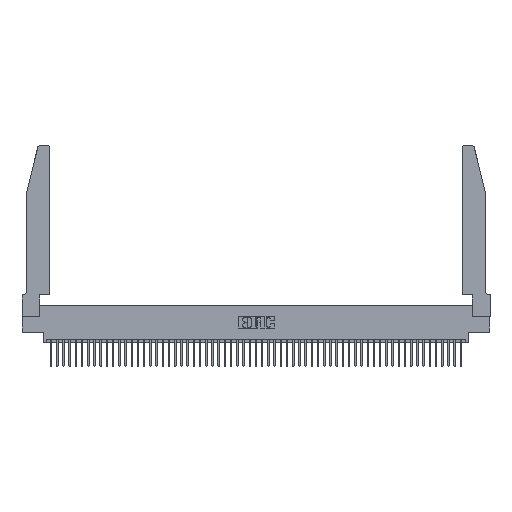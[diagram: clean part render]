
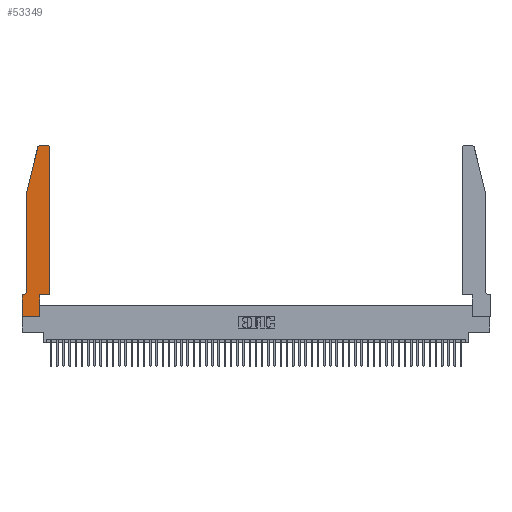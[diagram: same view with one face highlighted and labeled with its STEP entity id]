
A CAD part, top view. The second image highlights one B-rep face of the part: STEP entity #53349.
In plain terms, the highlighted planar face has unit normal (0, 0, 1).
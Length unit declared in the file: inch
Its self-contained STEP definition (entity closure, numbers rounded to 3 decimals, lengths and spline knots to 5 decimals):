
#798 = VECTOR ( 'NONE', #17286, 39.37008 ) ;
#1004 = LINE ( 'NONE', #35745, #33051 ) ;
#1583 = DIRECTION ( 'NONE',  ( -1., 0., 0. ) ) ;
#1916 = DIRECTION ( 'NONE',  ( -1., 0., 0. ) ) ;
#2500 = CARTESIAN_POINT ( 'NONE',  ( 0.4205, 2.72, 0.37 ) ) ;
#2625 = ORIENTED_EDGE ( 'NONE', *, *, #51947, .T. ) ;
#2763 = DIRECTION ( 'NONE',  ( 0., -1., 0. ) ) ;
#2934 = LINE ( 'NONE', #49160, #19914 ) ;
#3525 = VERTEX_POINT ( 'NONE', #50909 ) ;
#4084 = CARTESIAN_POINT ( 'NONE',  ( 0.4505, 0.35, 0.37 ) ) ;
#4349 = CARTESIAN_POINT ( 'NONE',  ( 0., 0., 0.37 ) ) ;
#5816 = VECTOR ( 'NONE', #54023, 39.37008 ) ;
#6450 = VERTEX_POINT ( 'NONE', #38576 ) ;
#6596 = CARTESIAN_POINT ( 'NONE',  ( 0., 0., 0.37 ) ) ;
#6844 = VERTEX_POINT ( 'NONE', #53510 ) ;
#7007 = VERTEX_POINT ( 'NONE', #29158 ) ;
#7315 = CARTESIAN_POINT ( 'NONE',  ( 0.0055, 0.35, 0.37 ) ) ;
#8256 = DIRECTION ( 'NONE',  ( 1., 0., 0. ) ) ;
#8524 = DIRECTION ( 'NONE',  ( 1., 0., 0. ) ) ;
#9118 = VECTOR ( 'NONE', #2763, 39.37008 ) ;
#9578 = PLANE ( 'NONE',  #10387 ) ;
#9923 = CARTESIAN_POINT ( 'NONE',  ( 0.0055, 0.42, 0.37 ) ) ;
#10387 = AXIS2_PLACEMENT_3D ( 'NONE', #50883, #25823, #30231 ) ;
#10836 = CARTESIAN_POINT ( 'NONE',  ( 0.4505, 0.35, 0.37 ) ) ;
#11260 = LINE ( 'NONE', #23453, #53171 ) ;
#11717 = CARTESIAN_POINT ( 'NONE',  ( 0.0755, 0.42, 0.37 ) ) ;
#12260 = CARTESIAN_POINT ( 'NONE',  ( 0.4505, 0.35, 0.37 ) ) ;
#13047 = CIRCLE ( 'NONE', #21134, 0.07 ) ;
#13954 = VERTEX_POINT ( 'NONE', #27053 ) ;
#17203 = LINE ( 'NONE', #29511, #798 ) ;
#17286 = DIRECTION ( 'NONE',  ( 0., -1., 0. ) ) ;
#18181 = VERTEX_POINT ( 'NONE', #27015 ) ;
#18691 = CARTESIAN_POINT ( 'NONE',  ( 0., 0.35, 0.37 ) ) ;
#18988 = ORIENTED_EDGE ( 'NONE', *, *, #26678, .T. ) ;
#19914 = VECTOR ( 'NONE', #27793, 39.37008 ) ;
#21134 = AXIS2_PLACEMENT_3D ( 'NONE', #9923, #26746, #1916 ) ;
#21680 = DIRECTION ( 'NONE',  ( 0., 0., 1. ) ) ;
#22556 = VERTEX_POINT ( 'NONE', #11717 ) ;
#22914 = DIRECTION ( 'NONE',  ( -1., 0., 0. ) ) ;
#23111 = VECTOR ( 'NONE', #8256, 39.37008 ) ;
#23453 = CARTESIAN_POINT ( 'NONE',  ( 0.2605, 2.75, 0.37 ) ) ;
#23586 = ORIENTED_EDGE ( 'NONE', *, *, #40031, .T. ) ;
#24282 = EDGE_CURVE ( 'NONE', #6844, #13954, #2934, .T. ) ;
#24577 = ORIENTED_EDGE ( 'NONE', *, *, #29394, .T. ) ;
#24908 = EDGE_CURVE ( 'NONE', #25732, #3525, #30283, .T. ) ;
#25732 = VERTEX_POINT ( 'NONE', #53954 ) ;
#25823 = DIRECTION ( 'NONE',  ( 0., 0., 1. ) ) ;
#25849 = DIRECTION ( 'NONE',  ( 1., 0., 0. ) ) ;
#26678 = EDGE_CURVE ( 'NONE', #6450, #6844, #50410, .T. ) ;
#26746 = DIRECTION ( 'NONE',  ( 0., 0., -1. ) ) ;
#26929 = DIRECTION ( 'NONE',  ( 0., 1., 0. ) ) ;
#27015 = CARTESIAN_POINT ( 'NONE',  ( 0.284, 2.75, 0.37 ) ) ;
#27053 = CARTESIAN_POINT ( 'NONE',  ( 0.2865, 0.35, 0.37 ) ) ;
#27793 = DIRECTION ( 'NONE',  ( 0., 1., 0. ) ) ;
#28003 = EDGE_CURVE ( 'NONE', #3525, #18181, #11260, .T. ) ;
#28181 = VERTEX_POINT ( 'NONE', #12260 ) ;
#28584 = EDGE_CURVE ( 'NONE', #40774, #6450, #43805, .T. ) ;
#29158 = CARTESIAN_POINT ( 'NONE',  ( 0.25487, 2.72718, 0.37 ) ) ;
#29394 = EDGE_CURVE ( 'NONE', #7007, #33338, #39862, .T. ) ;
#29511 = CARTESIAN_POINT ( 'NONE',  ( 0.0755, 2., 0.37 ) ) ;
#30231 = DIRECTION ( 'NONE',  ( 1., 0., 0. ) ) ;
#30283 = CIRCLE ( 'NONE', #42835, 0.03 ) ;
#33051 = VECTOR ( 'NONE', #1583, 39.37008 ) ;
#33338 = VERTEX_POINT ( 'NONE', #40072 ) ;
#34138 = ORIENTED_EDGE ( 'NONE', *, *, #24282, .T. ) ;
#34657 = ORIENTED_EDGE ( 'NONE', *, *, #24908, .T. ) ;
#35653 = CIRCLE ( 'NONE', #42200, 0.03 ) ;
#35744 = VECTOR ( 'NONE', #26929, 39.37008 ) ;
#35745 = CARTESIAN_POINT ( 'NONE',  ( 0.0755, 0.35, 0.37 ) ) ;
#36715 = EDGE_CURVE ( 'NONE', #22556, #51138, #13047, .T. ) ;
#37452 = ORIENTED_EDGE ( 'NONE', *, *, #43364, .T. ) ;
#38008 = EDGE_LOOP ( 'NONE', ( #42929, #23586, #24577, #47151, #41405, #37452, #41941, #18988, #34138, #2625, #48736, #34657 ) ) ;
#38576 = CARTESIAN_POINT ( 'NONE',  ( 0., 0., 0.37 ) ) ;
#38746 = EDGE_CURVE ( 'NONE', #28181, #25732, #53377, .T. ) ;
#39862 = LINE ( 'NONE', #49071, #5816 ) ;
#40031 = EDGE_CURVE ( 'NONE', #18181, #7007, #35653, .T. ) ;
#40072 = CARTESIAN_POINT ( 'NONE',  ( 0.0755, 2., 0.37 ) ) ;
#40774 = VERTEX_POINT ( 'NONE', #18691 ) ;
#41405 = ORIENTED_EDGE ( 'NONE', *, *, #36715, .T. ) ;
#41941 = ORIENTED_EDGE ( 'NONE', *, *, #28584, .T. ) ;
#41951 = VECTOR ( 'NONE', #8524, 39.37008 ) ;
#42200 = AXIS2_PLACEMENT_3D ( 'NONE', #46696, #21680, #25849 ) ;
#42835 = AXIS2_PLACEMENT_3D ( 'NONE', #2500, #52232, #44333 ) ;
#42929 = ORIENTED_EDGE ( 'NONE', *, *, #28003, .T. ) ;
#43364 = EDGE_CURVE ( 'NONE', #51138, #40774, #1004, .T. ) ;
#43366 = LINE ( 'NONE', #4084, #23111 ) ;
#43805 = LINE ( 'NONE', #6596, #9118 ) ;
#44333 = DIRECTION ( 'NONE',  ( 1., 0., 0. ) ) ;
#46696 = CARTESIAN_POINT ( 'NONE',  ( 0.284, 2.72, 0.37 ) ) ;
#47151 = ORIENTED_EDGE ( 'NONE', *, *, #47892, .T. ) ;
#47892 = EDGE_CURVE ( 'NONE', #33338, #22556, #17203, .T. ) ;
#48736 = ORIENTED_EDGE ( 'NONE', *, *, #38746, .T. ) ;
#49071 = CARTESIAN_POINT ( 'NONE',  ( 0.0755, 2., 0.37 ) ) ;
#49160 = CARTESIAN_POINT ( 'NONE',  ( 0.2865, 0.35, 0.37 ) ) ;
#50410 = LINE ( 'NONE', #4349, #41951 ) ;
#50883 = CARTESIAN_POINT ( 'NONE',  ( 0., 0.35, 0.37 ) ) ;
#50909 = CARTESIAN_POINT ( 'NONE',  ( 0.4205, 2.75, 0.37 ) ) ;
#51071 = FACE_OUTER_BOUND ( 'NONE', #38008, .T. ) ;
#51138 = VERTEX_POINT ( 'NONE', #7315 ) ;
#51947 = EDGE_CURVE ( 'NONE', #13954, #28181, #43366, .T. ) ;
#52232 = DIRECTION ( 'NONE',  ( 0., 0., 1. ) ) ;
#53171 = VECTOR ( 'NONE', #22914, 39.37008 ) ;
#53349 = ADVANCED_FACE ( 'NONE', ( #51071 ), #9578, .T. ) ;
#53377 = LINE ( 'NONE', #10836, #35744 ) ;
#53510 = CARTESIAN_POINT ( 'NONE',  ( 0.2865, 0., 0.37 ) ) ;
#53954 = CARTESIAN_POINT ( 'NONE',  ( 0.4505, 2.72, 0.37 ) ) ;
#54023 = DIRECTION ( 'NONE',  ( -0.239, -0.971, 0. ) ) ;
